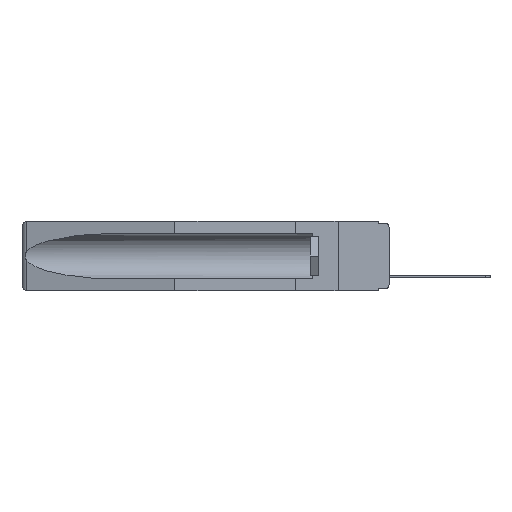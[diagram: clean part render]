
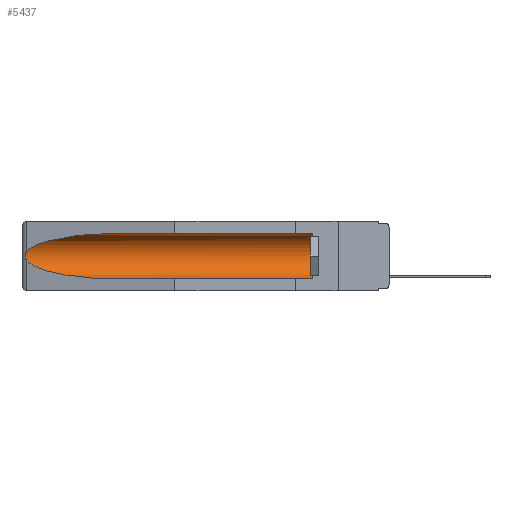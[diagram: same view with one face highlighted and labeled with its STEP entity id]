
A CAD part, left-side view. The second image highlights one B-rep face of the part: STEP entity #5437.
In plain terms, the highlighted cylindrical face has radius 2.857 mm (diameter 5.715 mm), a partial arc.
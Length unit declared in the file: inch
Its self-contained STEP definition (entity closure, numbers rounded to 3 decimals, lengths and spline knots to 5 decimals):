
#286 = EDGE_CURVE ( 'NONE', #3755, #11548, #15429, .T. ) ;
#299 = CARTESIAN_POINT ( 'NONE',  ( 0.155, 1.07973, -0.284 ) ) ;
#437 = CARTESIAN_POINT ( 'NONE',  ( 0.26597, 1.52961, -0.15275 ) ) ;
#520 = CARTESIAN_POINT ( 'NONE',  ( 0.26655, 1.53094, -0.18657 ) ) ;
#901 = VERTEX_POINT ( 'NONE', #22656 ) ;
#1293 = B_SPLINE_CURVE_WITH_KNOTS ( 'NONE', 3,
 ( #17117, #437, #9961, #6111, #13302, #13526, #9890, #520, #15372, #2340 ),
 .UNSPECIFIED., .F., .F.,
 ( 4, 2, 2, 2, 4 ),
 ( 0., 0.00029, 0.00058, 0.00087, 0.00117 ),
 .UNSPECIFIED. ) ;
#1594 = CARTESIAN_POINT ( 'NONE',  ( 0.26537, 1.52718, -0.19328 ) ) ;
#1927 = ORIENTED_EDGE ( 'NONE', *, *, #286, .T. ) ;
#2115 = VECTOR ( 'NONE', #3016, 39.37008 ) ;
#2279 = ORIENTED_EDGE ( 'NONE', *, *, #22776, .T. ) ;
#2340 = CARTESIAN_POINT ( 'NONE',  ( 0.26537, 1.52718, -0.19328 ) ) ;
#2438 = ORIENTED_EDGE ( 'NONE', *, *, #17319, .T. ) ;
#2457 = CYLINDRICAL_SURFACE ( 'NONE', #9637, 0.1125 ) ;
#2484 = CARTESIAN_POINT ( 'NONE',  ( 0.155, -0.30754, -0.059 ) ) ;
#3016 = DIRECTION ( 'NONE',  ( 0., 1., 0. ) ) ;
#3755 = VERTEX_POINT ( 'NONE', #21286 ) ;
#3803 = LINE ( 'NONE', #10417, #2115 ) ;
#3978 = LINE ( 'NONE', #2484, #22392 ) ;
#5437 = ADVANCED_FACE ( 'NONE', ( #20868 ), #2457, .F. ) ;
#6030 = ORIENTED_EDGE ( 'NONE', *, *, #9244, .T. ) ;
#6111 = CARTESIAN_POINT ( 'NONE',  ( 0.2673, 1.5327, -0.16383 ) ) ;
#6403 = ORIENTED_EDGE ( 'NONE', *, *, #9064, .T. ) ;
#7125 = CARTESIAN_POINT ( 'NONE',  ( 0.21114, 1.30732, -0.284 ) ) ;
#8709 = CARTESIAN_POINT ( 'NONE',  ( 0.155, -0.30754, -0.1715 ) ) ;
#9064 = EDGE_CURVE ( 'NONE', #14169, #901, #18346, .T. ) ;
#9153 = VERTEX_POINT ( 'NONE', #17721 ) ;
#9244 = EDGE_CURVE ( 'NONE', #9153, #12429, #17608, .T. ) ;
#9637 = AXIS2_PLACEMENT_3D ( 'NONE', #8709, #21877, #10630 ) ;
#9890 = CARTESIAN_POINT ( 'NONE',  ( 0.2673, 1.53269, -0.17917 ) ) ;
#9961 = CARTESIAN_POINT ( 'NONE',  ( 0.26654, 1.53092, -0.15636 ) ) ;
#10242 = CARTESIAN_POINT ( 'NONE',  ( 0.155, 0.126, -0.1715 ) ) ;
#10417 = CARTESIAN_POINT ( 'NONE',  ( 0.155, -0.30754, -0.284 ) ) ;
#10630 = DIRECTION ( 'NONE',  ( 0., 0., 1. ) ) ;
#11480 = EDGE_CURVE ( 'NONE', #14169, #12429, #3803, .T. ) ;
#11548 = VERTEX_POINT ( 'NONE', #12370 ) ;
#12234 = CARTESIAN_POINT ( 'NONE',  ( 0.155, 1.07973, -0.059 ) ) ;
#12370 = CARTESIAN_POINT ( 'NONE',  ( 0.26537, 1.52718, -0.14972 ) ) ;
#12429 = VERTEX_POINT ( 'NONE', #299 ) ;
#12647 = CARTESIAN_POINT ( 'NONE',  ( 0.25451, 1.48313, -0.09465 ) ) ;
#13302 = CARTESIAN_POINT ( 'NONE',  ( 0.2675, 1.53308, -0.16763 ) ) ;
#13526 = CARTESIAN_POINT ( 'NONE',  ( 0.2675, 1.53308, -0.17534 ) ) ;
#13750 = DIRECTION ( 'NONE',  ( 0., 0., 1. ) ) ;
#14103 = CARTESIAN_POINT ( 'NONE',  ( 0.21114, 1.30732, -0.059 ) ) ;
#14169 = VERTEX_POINT ( 'NONE', #15856 ) ;
#15372 = CARTESIAN_POINT ( 'NONE',  ( 0.26597, 1.5296, -0.19026 ) ) ;
#15429 =( BOUNDED_CURVE ( )  B_SPLINE_CURVE ( 3, ( #12234, #14103, #12647, #21856 ),
 .UNSPECIFIED., .F., .F. ) 
 B_SPLINE_CURVE_WITH_KNOTS ( ( 4, 4 ),
 ( 4.71239, 6.08839 ),
 .UNSPECIFIED. ) 
 CURVE ( )  GEOMETRIC_REPRESENTATION_ITEM ( )  RATIONAL_B_SPLINE_CURVE ( ( 1., 0.848, 0.848, 1. ) ) 
 REPRESENTATION_ITEM ( '' )  );
#15540 = AXIS2_PLACEMENT_3D ( 'NONE', #10242, #15740, #13750 ) ;
#15740 = DIRECTION ( 'NONE',  ( 0., -1., 0. ) ) ;
#15856 = CARTESIAN_POINT ( 'NONE',  ( 0.155, 0.126, -0.284 ) ) ;
#17117 = CARTESIAN_POINT ( 'NONE',  ( 0.26537, 1.52718, -0.14972 ) ) ;
#17319 = EDGE_CURVE ( 'NONE', #901, #3755, #3978, .T. ) ;
#17608 =( BOUNDED_CURVE ( )  B_SPLINE_CURVE ( 3, ( #1594, #23415, #7125, #17805 ),
 .UNSPECIFIED., .F., .F. ) 
 B_SPLINE_CURVE_WITH_KNOTS ( ( 4, 4 ),
 ( 0.1948, 1.5708 ),
 .UNSPECIFIED. ) 
 CURVE ( )  GEOMETRIC_REPRESENTATION_ITEM ( )  RATIONAL_B_SPLINE_CURVE ( ( 1., 0.848, 0.848, 1. ) ) 
 REPRESENTATION_ITEM ( '' )  );
#17721 = CARTESIAN_POINT ( 'NONE',  ( 0.26537, 1.52718, -0.19328 ) ) ;
#17805 = CARTESIAN_POINT ( 'NONE',  ( 0.155, 1.07973, -0.284 ) ) ;
#18346 = CIRCLE ( 'NONE', #15540, 0.1125 ) ;
#19992 = EDGE_LOOP ( 'NONE', ( #1927, #2279, #6030, #20734, #6403, #2438 ) ) ;
#20734 = ORIENTED_EDGE ( 'NONE', *, *, #11480, .F. ) ;
#20868 = FACE_OUTER_BOUND ( 'NONE', #19992, .T. ) ;
#21286 = CARTESIAN_POINT ( 'NONE',  ( 0.155, 1.07973, -0.059 ) ) ;
#21856 = CARTESIAN_POINT ( 'NONE',  ( 0.26537, 1.52718, -0.14972 ) ) ;
#21877 = DIRECTION ( 'NONE',  ( 0., 1., 0. ) ) ;
#22392 = VECTOR ( 'NONE', #22898, 39.37008 ) ;
#22656 = CARTESIAN_POINT ( 'NONE',  ( 0.155, 0.126, -0.059 ) ) ;
#22776 = EDGE_CURVE ( 'NONE', #11548, #9153, #1293, .T. ) ;
#22898 = DIRECTION ( 'NONE',  ( 0., 1., 0. ) ) ;
#23415 = CARTESIAN_POINT ( 'NONE',  ( 0.25451, 1.48313, -0.24835 ) ) ;
